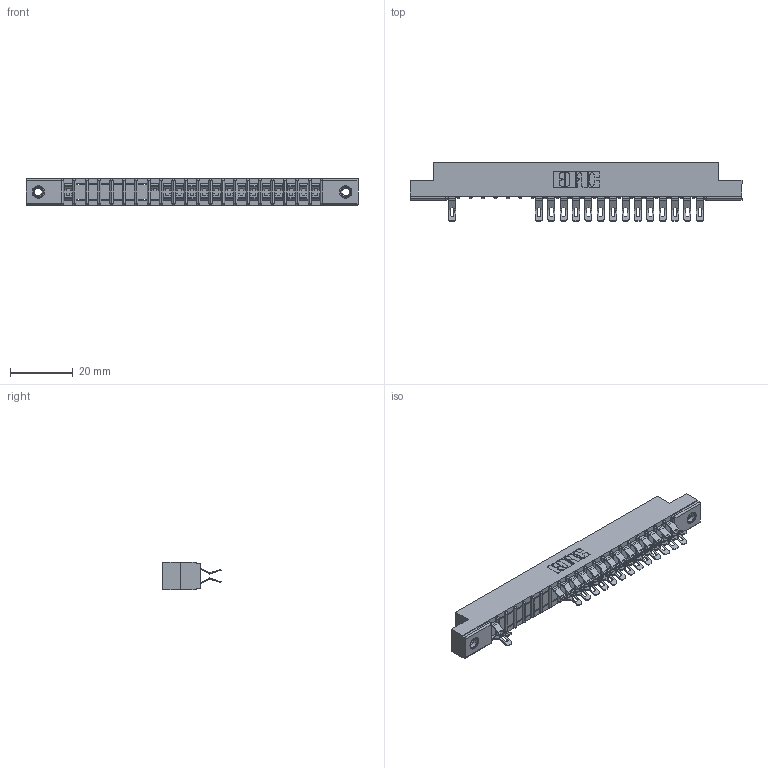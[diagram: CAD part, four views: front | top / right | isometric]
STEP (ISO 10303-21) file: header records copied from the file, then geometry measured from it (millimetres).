
FILE_DESCRIPTION (( 'STEP AP203' ), '1' );
FILE_NAME ('307-042-555-207.STEP', '2018-08-05T18:25:16', ( '' ), ( '' ), 'SwSTEP 2.0', 'SolidWorks 2016', '' );
FILE_SCHEMA (( 'CONFIG_CONTROL_DESIGN' ));
Length unit declared in the file: inch
Products named in the file (4): 307-042-555-207; 307 Part_.156 Dia Mounting Holes; 307-290-001_555; 345-250-001_345-250-005-103
Assembly tree (32 placements, depth 2):
  307-042-555-207
    307 Part_.156 Dia Mounting Holes
    307-290-001_555  x29
    345-250-001_345-250-005-103  x2
Bounding box: 106.22 x 18.75 x 8.71 mm (x, y, z)
Volume: 6852.8 mm3; surface area: 11572.9 mm2
Topology: 32 solids, 32 shells, 2099 faces, 6124 edges, 3976 vertices
Faces by surface type: plane 1166, cylinder 873, sphere 44, cone 12, torus 4
Entity records: 22570 total; most frequent: CARTESIAN_POINT 3743, ORIENTED_EDGE 3716, DIRECTION 3678, EDGE_CURVE 1858, LINE 1404, VECTOR 1404, VERTEX_POINT 1202, AXIS2_PLACEMENT_3D 1137
